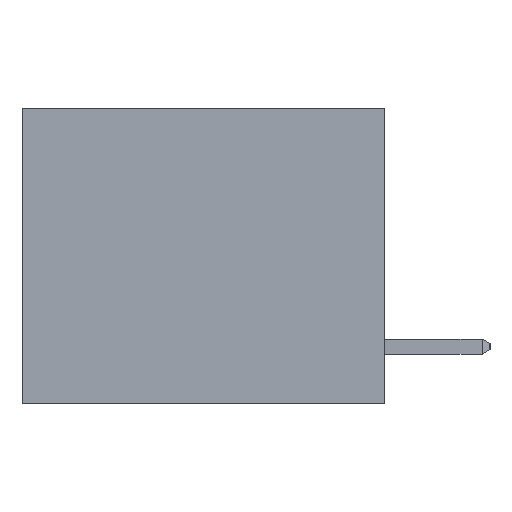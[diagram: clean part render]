
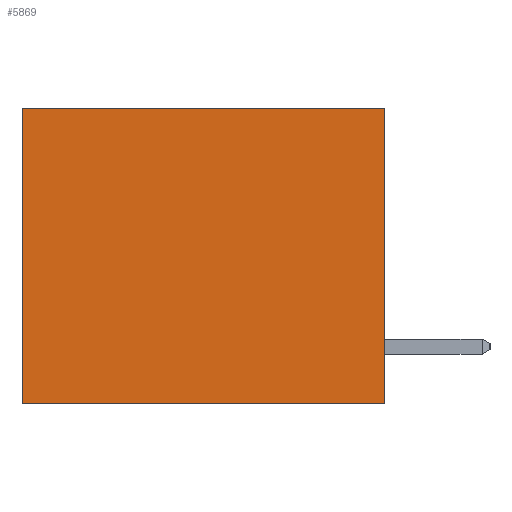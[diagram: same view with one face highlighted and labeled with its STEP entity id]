
A CAD part, left-side view. The second image highlights one B-rep face of the part: STEP entity #5869.
In plain terms, the highlighted planar face has unit normal (-1, 0, 0).
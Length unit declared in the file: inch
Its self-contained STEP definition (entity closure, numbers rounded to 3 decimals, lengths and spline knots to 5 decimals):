
#328 = DIRECTION ( 'NONE',  ( 0., 1., 0. ) ) ;
#403 = CARTESIAN_POINT ( 'NONE',  ( 0.3165, 0.6, -0.49 ) ) ;
#532 = VERTEX_POINT ( 'NONE', #29280 ) ;
#844 = VERTEX_POINT ( 'NONE', #14580 ) ;
#1368 = ORIENTED_EDGE ( 'NONE', *, *, #18301, .T. ) ;
#2456 = ORIENTED_EDGE ( 'NONE', *, *, #18883, .F. ) ;
#2689 = LINE ( 'NONE', #27306, #26738 ) ;
#2809 = LINE ( 'NONE', #9403, #6586 ) ;
#4104 = VECTOR ( 'NONE', #29362, 39.37008 ) ;
#5869 = ADVANCED_FACE ( 'NONE', ( #28328 ), #7119, .F. ) ;
#6586 = VECTOR ( 'NONE', #20915, 39.37008 ) ;
#7010 = VECTOR ( 'NONE', #15729, 39.37008 ) ;
#7119 = PLANE ( 'NONE',  #10000 ) ;
#8152 = LINE ( 'NONE', #30442, #7010 ) ;
#8324 = CARTESIAN_POINT ( 'NONE',  ( 0.3165, 0., 0. ) ) ;
#9403 = CARTESIAN_POINT ( 'NONE',  ( 0.3165, 0., -0.49 ) ) ;
#10000 = AXIS2_PLACEMENT_3D ( 'NONE', #14988, #12800, #15096 ) ;
#10274 = VERTEX_POINT ( 'NONE', #25833 ) ;
#12800 = DIRECTION ( 'NONE',  ( 1., 0., 0. ) ) ;
#14481 = ORIENTED_EDGE ( 'NONE', *, *, #30990, .T. ) ;
#14580 = CARTESIAN_POINT ( 'NONE',  ( 0.3165, 0., -0.49 ) ) ;
#14988 = CARTESIAN_POINT ( 'NONE',  ( 0.3165, 0., -0.49 ) ) ;
#15096 = DIRECTION ( 'NONE',  ( 0., 0., -1. ) ) ;
#15381 = EDGE_CURVE ( 'NONE', #844, #532, #2689, .T. ) ;
#15729 = DIRECTION ( 'NONE',  ( 0., 1., 0. ) ) ;
#18301 = EDGE_CURVE ( 'NONE', #26317, #10274, #8152, .T. ) ;
#18883 = EDGE_CURVE ( 'NONE', #26317, #844, #2809, .T. ) ;
#20915 = DIRECTION ( 'NONE',  ( 0., 0., -1. ) ) ;
#21340 = LINE ( 'NONE', #403, #4104 ) ;
#25833 = CARTESIAN_POINT ( 'NONE',  ( 0.3165, 0.6, 0. ) ) ;
#25870 = ORIENTED_EDGE ( 'NONE', *, *, #15381, .F. ) ;
#26317 = VERTEX_POINT ( 'NONE', #8324 ) ;
#26738 = VECTOR ( 'NONE', #328, 39.37008 ) ;
#27306 = CARTESIAN_POINT ( 'NONE',  ( 0.3165, 0., -0.49 ) ) ;
#28125 = EDGE_LOOP ( 'NONE', ( #14481, #25870, #2456, #1368 ) ) ;
#28328 = FACE_OUTER_BOUND ( 'NONE', #28125, .T. ) ;
#29280 = CARTESIAN_POINT ( 'NONE',  ( 0.3165, 0.6, -0.49 ) ) ;
#29362 = DIRECTION ( 'NONE',  ( 0., 0., -1. ) ) ;
#30442 = CARTESIAN_POINT ( 'NONE',  ( 0.3165, 0., 0. ) ) ;
#30990 = EDGE_CURVE ( 'NONE', #10274, #532, #21340, .T. ) ;
